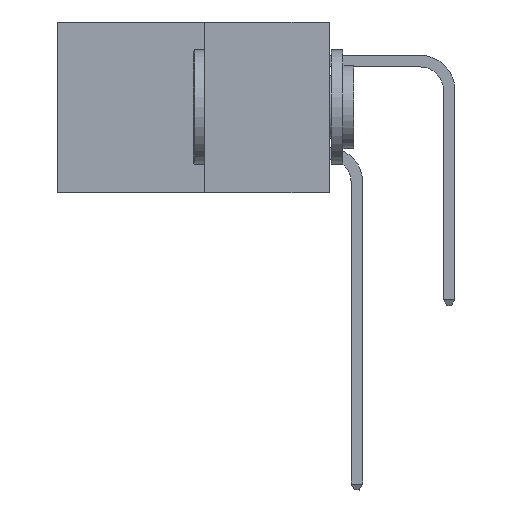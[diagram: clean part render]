
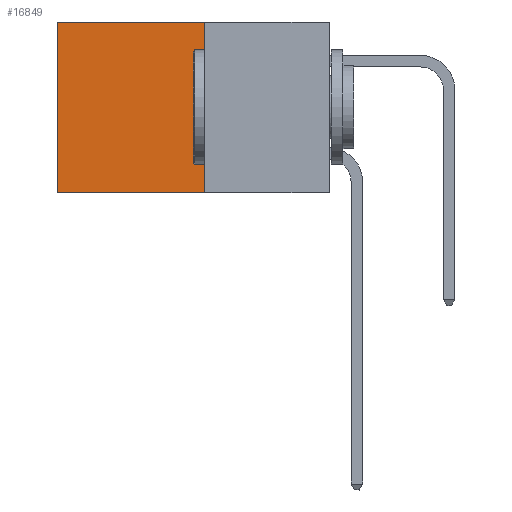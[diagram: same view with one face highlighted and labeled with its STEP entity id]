
A CAD part, left-side view. The second image highlights one B-rep face of the part: STEP entity #16849.
In plain terms, the highlighted planar face has unit normal (-1, 0, 0).
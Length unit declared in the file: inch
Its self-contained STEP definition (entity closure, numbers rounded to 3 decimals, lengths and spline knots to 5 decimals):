
#255 = CARTESIAN_POINT ( 'NONE',  ( 0.277, 0.27, 0. ) ) ;
#2370 = ORIENTED_EDGE ( 'NONE', *, *, #6750, .F. ) ;
#2449 = VERTEX_POINT ( 'NONE', #23995 ) ;
#2715 = EDGE_CURVE ( 'NONE', #21057, #2449, #9725, .T. ) ;
#5734 = DIRECTION ( 'NONE',  ( 0., 0., -1. ) ) ;
#5857 = EDGE_CURVE ( 'NONE', #2449, #9346, #7015, .T. ) ;
#6750 = EDGE_CURVE ( 'NONE', #21057, #7459, #24697, .T. ) ;
#6822 = CARTESIAN_POINT ( 'NONE',  ( 0.277, 0.27, -0.37 ) ) ;
#7015 = LINE ( 'NONE', #11060, #7672 ) ;
#7459 = VERTEX_POINT ( 'NONE', #6822 ) ;
#7623 = VECTOR ( 'NONE', #20468, 39.37008 ) ;
#7672 = VECTOR ( 'NONE', #11273, 39.37008 ) ;
#9346 = VERTEX_POINT ( 'NONE', #12881 ) ;
#9725 = LINE ( 'NONE', #255, #15539 ) ;
#10284 = ORIENTED_EDGE ( 'NONE', *, *, #2715, .T. ) ;
#10945 = VECTOR ( 'NONE', #24280, 39.37008 ) ;
#11060 = CARTESIAN_POINT ( 'NONE',  ( 0.277, 0.59, -0.37 ) ) ;
#11273 = DIRECTION ( 'NONE',  ( 0., 0., -1. ) ) ;
#11633 = LINE ( 'NONE', #22163, #10945 ) ;
#12881 = CARTESIAN_POINT ( 'NONE',  ( 0.277, 0.59, -0.37 ) ) ;
#14387 = PLANE ( 'NONE',  #18257 ) ;
#14578 = ORIENTED_EDGE ( 'NONE', *, *, #5857, .T. ) ;
#15539 = VECTOR ( 'NONE', #23873, 39.37008 ) ;
#15968 = CARTESIAN_POINT ( 'NONE',  ( 0.277, 0.27, -0.37 ) ) ;
#16600 = EDGE_LOOP ( 'NONE', ( #14578, #25185, #2370, #10284 ) ) ;
#16849 = ADVANCED_FACE ( 'NONE', ( #20928 ), #14387, .F. ) ;
#18257 = AXIS2_PLACEMENT_3D ( 'NONE', #24797, #18662, #5734 ) ;
#18662 = DIRECTION ( 'NONE',  ( 1., 0., 0. ) ) ;
#20468 = DIRECTION ( 'NONE',  ( 0., 0., -1. ) ) ;
#20928 = FACE_OUTER_BOUND ( 'NONE', #16600, .T. ) ;
#21057 = VERTEX_POINT ( 'NONE', #26362 ) ;
#22163 = CARTESIAN_POINT ( 'NONE',  ( 0.277, 0.27, -0.37 ) ) ;
#22320 = EDGE_CURVE ( 'NONE', #7459, #9346, #11633, .T. ) ;
#23873 = DIRECTION ( 'NONE',  ( 0., 1., 0. ) ) ;
#23995 = CARTESIAN_POINT ( 'NONE',  ( 0.277, 0.59, 0. ) ) ;
#24280 = DIRECTION ( 'NONE',  ( 0., 1., 0. ) ) ;
#24697 = LINE ( 'NONE', #15968, #7623 ) ;
#24797 = CARTESIAN_POINT ( 'NONE',  ( 0.277, 0.27, -0.37 ) ) ;
#25185 = ORIENTED_EDGE ( 'NONE', *, *, #22320, .F. ) ;
#26362 = CARTESIAN_POINT ( 'NONE',  ( 0.277, 0.27, 0. ) ) ;
